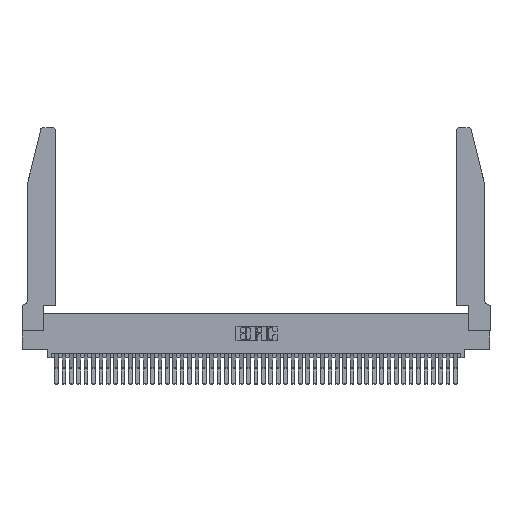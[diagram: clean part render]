
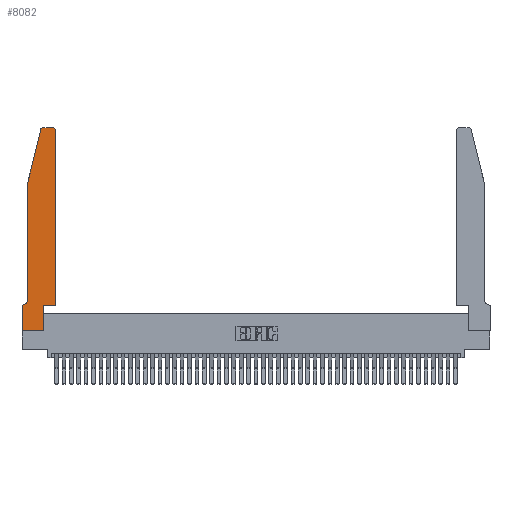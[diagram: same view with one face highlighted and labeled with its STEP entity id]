
A CAD part, top view. The second image highlights one B-rep face of the part: STEP entity #8082.
In plain terms, the highlighted planar face has unit normal (0, 0, 1).
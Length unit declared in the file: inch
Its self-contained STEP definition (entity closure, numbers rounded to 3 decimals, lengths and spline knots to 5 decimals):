
#342 = ORIENTED_EDGE ( 'NONE', *, *, #5336, .T. ) ;
#2121 = EDGE_CURVE ( 'NONE', #25708, #17736, #28869, .T. ) ;
#2390 = CARTESIAN_POINT ( 'NONE',  ( 0.4205, 2.72, 0.37 ) ) ;
#2444 = VECTOR ( 'NONE', #19158, 39.37008 ) ;
#2597 = EDGE_CURVE ( 'NONE', #17187, #6180, #28822, .T. ) ;
#3741 = AXIS2_PLACEMENT_3D ( 'NONE', #2390, #27565, #6040 ) ;
#5336 = EDGE_CURVE ( 'NONE', #17736, #17187, #35330, .T. ) ;
#5559 = EDGE_CURVE ( 'NONE', #22709, #28680, #16939, .T. ) ;
#6040 = DIRECTION ( 'NONE',  ( 1., 0., 0. ) ) ;
#6180 = VERTEX_POINT ( 'NONE', #25593 ) ;
#7735 = CARTESIAN_POINT ( 'NONE',  ( 0.4505, 2.72, 0.37 ) ) ;
#8082 = ADVANCED_FACE ( 'NONE', ( #26765 ), #28877, .T. ) ;
#8101 = DIRECTION ( 'NONE',  ( 0., -1., 0. ) ) ;
#9438 = DIRECTION ( 'NONE',  ( -1., 0., 0. ) ) ;
#9548 = DIRECTION ( 'NONE',  ( 0., 0., 1. ) ) ;
#9986 = VERTEX_POINT ( 'NONE', #7735 ) ;
#10448 = CARTESIAN_POINT ( 'NONE',  ( 0., 0., 0.37 ) ) ;
#11187 = EDGE_CURVE ( 'NONE', #33099, #38876, #35339, .T. ) ;
#13443 = CARTESIAN_POINT ( 'NONE',  ( 0.2865, 0.35, 0.37 ) ) ;
#13689 = VERTEX_POINT ( 'NONE', #27858 ) ;
#13784 = VECTOR ( 'NONE', #40580, 39.37008 ) ;
#15976 = DIRECTION ( 'NONE',  ( -0.239, -0.971, 0. ) ) ;
#16292 = ORIENTED_EDGE ( 'NONE', *, *, #2597, .T. ) ;
#16400 = VECTOR ( 'NONE', #15976, 39.37008 ) ;
#16939 = LINE ( 'NONE', #13443, #44184 ) ;
#17187 = VERTEX_POINT ( 'NONE', #24754 ) ;
#17736 = VERTEX_POINT ( 'NONE', #42072 ) ;
#18276 = DIRECTION ( 'NONE',  ( 0., 0., 1. ) ) ;
#18560 = CARTESIAN_POINT ( 'NONE',  ( 0., 0.35, 0.37 ) ) ;
#19158 = DIRECTION ( 'NONE',  ( 0., 1., 0. ) ) ;
#19357 = VECTOR ( 'NONE', #8101, 39.37008 ) ;
#19620 = CARTESIAN_POINT ( 'NONE',  ( 0.2865, 0.35, 0.37 ) ) ;
#19669 = ORIENTED_EDGE ( 'NONE', *, *, #33130, .T. ) ;
#19912 = EDGE_CURVE ( 'NONE', #38876, #43452, #20891, .T. ) ;
#20891 = LINE ( 'NONE', #10448, #44768 ) ;
#21532 = ORIENTED_EDGE ( 'NONE', *, *, #26741, .T. ) ;
#22709 = VERTEX_POINT ( 'NONE', #32862 ) ;
#24288 = AXIS2_PLACEMENT_3D ( 'NONE', #31020, #9548, #34561 ) ;
#24754 = CARTESIAN_POINT ( 'NONE',  ( 0.0755, 2., 0.37 ) ) ;
#25593 = CARTESIAN_POINT ( 'NONE',  ( 0.0755, 0.42, 0.37 ) ) ;
#25670 = CARTESIAN_POINT ( 'NONE',  ( 0.0755, 0.35, 0.37 ) ) ;
#25708 = VERTEX_POINT ( 'NONE', #26880 ) ;
#25914 = VECTOR ( 'NONE', #32826, 39.37008 ) ;
#26741 = EDGE_CURVE ( 'NONE', #33018, #9986, #39406, .T. ) ;
#26765 = FACE_OUTER_BOUND ( 'NONE', #31689, .T. ) ;
#26841 = AXIS2_PLACEMENT_3D ( 'NONE', #39555, #18276, #43111 ) ;
#26880 = CARTESIAN_POINT ( 'NONE',  ( 0.284, 2.75, 0.37 ) ) ;
#26945 = LINE ( 'NONE', #42171, #35260 ) ;
#27322 = CARTESIAN_POINT ( 'NONE',  ( 0.2605, 2.75, 0.37 ) ) ;
#27565 = DIRECTION ( 'NONE',  ( 0., 0., 1. ) ) ;
#27649 = AXIS2_PLACEMENT_3D ( 'NONE', #34185, #41506, #41497 ) ;
#27858 = CARTESIAN_POINT ( 'NONE',  ( 0.4205, 2.75, 0.37 ) ) ;
#28392 = ORIENTED_EDGE ( 'NONE', *, *, #5559, .T. ) ;
#28680 = VERTEX_POINT ( 'NONE', #19620 ) ;
#28822 = LINE ( 'NONE', #43645, #19357 ) ;
#28869 = CIRCLE ( 'NONE', #24288, 0.03 ) ;
#28877 = PLANE ( 'NONE',  #26841 ) ;
#28948 = CARTESIAN_POINT ( 'NONE',  ( 0., 0., 0.37 ) ) ;
#29824 = ORIENTED_EDGE ( 'NONE', *, *, #19912, .T. ) ;
#30494 = CARTESIAN_POINT ( 'NONE',  ( 0.0055, 0.35, 0.37 ) ) ;
#31020 = CARTESIAN_POINT ( 'NONE',  ( 0.284, 2.72, 0.37 ) ) ;
#31689 = EDGE_LOOP ( 'NONE', ( #44618, #31898, #342, #16292, #19669, #32233, #29824, #37179, #28392, #31761, #21532, #39336 ) ) ;
#31761 = ORIENTED_EDGE ( 'NONE', *, *, #38591, .T. ) ;
#31898 = ORIENTED_EDGE ( 'NONE', *, *, #2121, .T. ) ;
#32233 = ORIENTED_EDGE ( 'NONE', *, *, #11187, .T. ) ;
#32380 = EDGE_CURVE ( 'NONE', #43452, #22709, #42173, .T. ) ;
#32826 = DIRECTION ( 'NONE',  ( -1., 0., 0. ) ) ;
#32862 = CARTESIAN_POINT ( 'NONE',  ( 0.2865, 0., 0.37 ) ) ;
#33018 = VERTEX_POINT ( 'NONE', #40525 ) ;
#33099 = VERTEX_POINT ( 'NONE', #30494 ) ;
#33130 = EDGE_CURVE ( 'NONE', #6180, #33099, #37772, .T. ) ;
#34185 = CARTESIAN_POINT ( 'NONE',  ( 0.0055, 0.42, 0.37 ) ) ;
#34561 = DIRECTION ( 'NONE',  ( 1., 0., 0. ) ) ;
#35260 = VECTOR ( 'NONE', #38606, 39.37008 ) ;
#35330 = LINE ( 'NONE', #37305, #16400 ) ;
#35339 = LINE ( 'NONE', #25670, #25914 ) ;
#37019 = CARTESIAN_POINT ( 'NONE',  ( 0., 0., 0.37 ) ) ;
#37179 = ORIENTED_EDGE ( 'NONE', *, *, #32380, .T. ) ;
#37305 = CARTESIAN_POINT ( 'NONE',  ( 0.0755, 2., 0.37 ) ) ;
#37772 = CIRCLE ( 'NONE', #27649, 0.07 ) ;
#38363 = DIRECTION ( 'NONE',  ( 0., 1., 0. ) ) ;
#38591 = EDGE_CURVE ( 'NONE', #28680, #33018, #26945, .T. ) ;
#38606 = DIRECTION ( 'NONE',  ( 1., 0., 0. ) ) ;
#38876 = VERTEX_POINT ( 'NONE', #18560 ) ;
#39336 = ORIENTED_EDGE ( 'NONE', *, *, #41132, .T. ) ;
#39406 = LINE ( 'NONE', #44003, #2444 ) ;
#39555 = CARTESIAN_POINT ( 'NONE',  ( 0., 0.35, 0.37 ) ) ;
#40064 = VECTOR ( 'NONE', #9438, 39.37008 ) ;
#40440 = EDGE_CURVE ( 'NONE', #13689, #25708, #42274, .T. ) ;
#40525 = CARTESIAN_POINT ( 'NONE',  ( 0.4505, 0.35, 0.37 ) ) ;
#40555 = CIRCLE ( 'NONE', #3741, 0.03 ) ;
#40580 = DIRECTION ( 'NONE',  ( 1., 0., 0. ) ) ;
#41132 = EDGE_CURVE ( 'NONE', #9986, #13689, #40555, .T. ) ;
#41497 = DIRECTION ( 'NONE',  ( -1., 0., 0. ) ) ;
#41506 = DIRECTION ( 'NONE',  ( 0., 0., -1. ) ) ;
#42072 = CARTESIAN_POINT ( 'NONE',  ( 0.25487, 2.72718, 0.37 ) ) ;
#42171 = CARTESIAN_POINT ( 'NONE',  ( 0.4505, 0.35, 0.37 ) ) ;
#42173 = LINE ( 'NONE', #37019, #13784 ) ;
#42274 = LINE ( 'NONE', #27322, #40064 ) ;
#43111 = DIRECTION ( 'NONE',  ( 1., 0., 0. ) ) ;
#43452 = VERTEX_POINT ( 'NONE', #28948 ) ;
#43645 = CARTESIAN_POINT ( 'NONE',  ( 0.0755, 2., 0.37 ) ) ;
#44003 = CARTESIAN_POINT ( 'NONE',  ( 0.4505, 0.35, 0.37 ) ) ;
#44184 = VECTOR ( 'NONE', #38363, 39.37008 ) ;
#44618 = ORIENTED_EDGE ( 'NONE', *, *, #40440, .T. ) ;
#44768 = VECTOR ( 'NONE', #46115, 39.37008 ) ;
#46115 = DIRECTION ( 'NONE',  ( 0., -1., 0. ) ) ;
